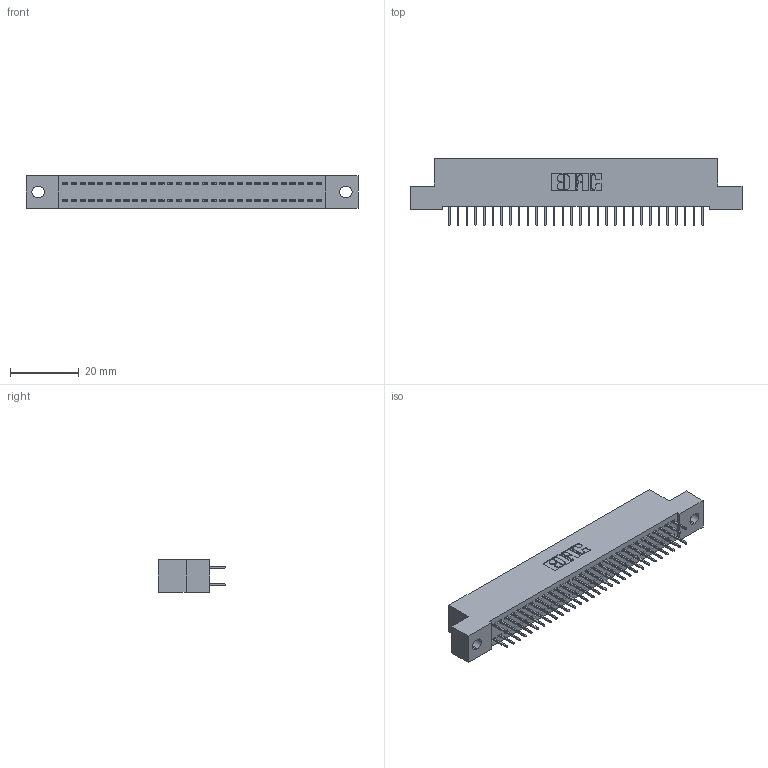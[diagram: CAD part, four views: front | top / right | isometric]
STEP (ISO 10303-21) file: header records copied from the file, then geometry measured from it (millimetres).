
FILE_DESCRIPTION (( 'STEP AP203' ), '1' );
FILE_NAME ('342-060-524-202.STEP', '2019-10-03T13:20:19', ( '' ), ( '' ), 'SwSTEP 2.0', 'SolidWorks 2016', '' );
FILE_SCHEMA (( 'CONFIG_CONTROL_DESIGN' ));
Length unit declared in the file: inch
Products named in the file (3): 342-060-524-202; 342 Part_.128 Slot; 345-292-001_345-293-124
Assembly tree (61 placements, depth 2):
  342-060-524-202
    342 Part_.128 Slot
    345-292-001_345-293-124  x60
Bounding box: 96.52 x 19.69 x 9.4 mm (x, y, z)
Volume: 8472.6 mm3; surface area: 13018.8 mm2
Topology: 61 solids, 61 shells, 3474 faces, 9851 edges, 6326 vertices
Faces by surface type: plane 2590, cylinder 884
Entity records: 20929 total; most frequent: CARTESIAN_POINT 3482, ORIENTED_EDGE 3418, DIRECTION 2997, EDGE_CURVE 1709, LINE 1585, VECTOR 1585, VERTEX_POINT 1134, AXIS2_PLACEMENT_3D 706
